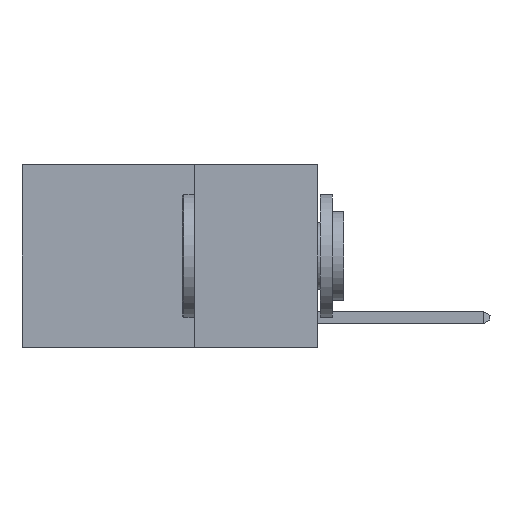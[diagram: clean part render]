
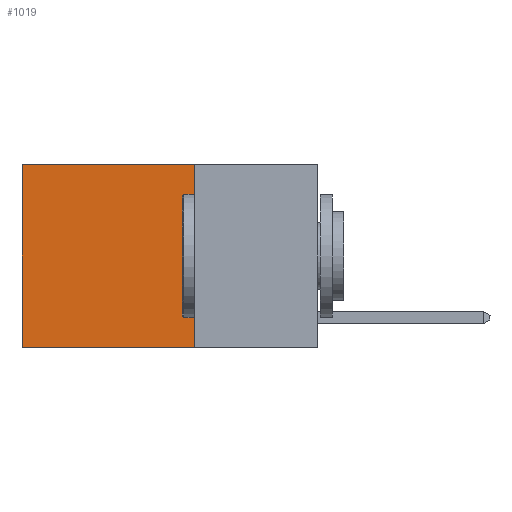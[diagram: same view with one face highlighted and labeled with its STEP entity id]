
A CAD part, left-side view. The second image highlights one B-rep face of the part: STEP entity #1019.
In plain terms, the highlighted planar face has unit normal (-1, 0, 0).
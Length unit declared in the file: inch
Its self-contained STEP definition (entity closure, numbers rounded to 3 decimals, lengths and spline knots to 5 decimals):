
#1019 = ADVANCED_FACE ( 'NONE', ( #9608 ), #25458, .F. ) ;
#2523 = VERTEX_POINT ( 'NONE', #10517 ) ;
#2994 = VECTOR ( 'NONE', #6338, 39.37008 ) ;
#3358 = AXIS2_PLACEMENT_3D ( 'NONE', #23123, #21051, #21425 ) ;
#3400 = LINE ( 'NONE', #19152, #12625 ) ;
#4655 = CARTESIAN_POINT ( 'NONE',  ( 0.2625, 0.25, 0. ) ) ;
#4751 = CARTESIAN_POINT ( 'NONE',  ( 0.2625, 0.6, 0. ) ) ;
#6338 = DIRECTION ( 'NONE',  ( 0., 1., 0. ) ) ;
#6712 = LINE ( 'NONE', #24162, #2994 ) ;
#6825 = DIRECTION ( 'NONE',  ( 0., 0., -1. ) ) ;
#8921 = VERTEX_POINT ( 'NONE', #10152 ) ;
#9272 = DIRECTION ( 'NONE',  ( 0., 0., -1. ) ) ;
#9608 = FACE_OUTER_BOUND ( 'NONE', #25697, .T. ) ;
#10152 = CARTESIAN_POINT ( 'NONE',  ( 0.2625, 0.6, -0.37 ) ) ;
#10384 = ORIENTED_EDGE ( 'NONE', *, *, #19988, .F. ) ;
#10517 = CARTESIAN_POINT ( 'NONE',  ( 0.2625, 0.6, 0. ) ) ;
#11798 = VECTOR ( 'NONE', #22477, 39.37008 ) ;
#12625 = VECTOR ( 'NONE', #9272, 39.37008 ) ;
#12741 = LINE ( 'NONE', #4655, #11798 ) ;
#12974 = EDGE_CURVE ( 'NONE', #18707, #8921, #6712, .T. ) ;
#14227 = ORIENTED_EDGE ( 'NONE', *, *, #12974, .F. ) ;
#14726 = CARTESIAN_POINT ( 'NONE',  ( 0.2625, 0.25, 0. ) ) ;
#17532 = EDGE_CURVE ( 'NONE', #22972, #2523, #12741, .T. ) ;
#18707 = VERTEX_POINT ( 'NONE', #22540 ) ;
#19152 = CARTESIAN_POINT ( 'NONE',  ( 0.2625, 0.25, 0. ) ) ;
#19363 = EDGE_CURVE ( 'NONE', #2523, #8921, #24150, .T. ) ;
#19988 = EDGE_CURVE ( 'NONE', #22972, #18707, #3400, .T. ) ;
#20817 = ORIENTED_EDGE ( 'NONE', *, *, #17532, .T. ) ;
#21051 = DIRECTION ( 'NONE',  ( 1., 0., 0. ) ) ;
#21425 = DIRECTION ( 'NONE',  ( 0., 0., -1. ) ) ;
#22477 = DIRECTION ( 'NONE',  ( 0., 1., 0. ) ) ;
#22540 = CARTESIAN_POINT ( 'NONE',  ( 0.2625, 0.25, -0.37 ) ) ;
#22957 = VECTOR ( 'NONE', #6825, 39.37008 ) ;
#22972 = VERTEX_POINT ( 'NONE', #14726 ) ;
#23123 = CARTESIAN_POINT ( 'NONE',  ( 0.2625, 0.25, 0. ) ) ;
#24150 = LINE ( 'NONE', #4751, #22957 ) ;
#24162 = CARTESIAN_POINT ( 'NONE',  ( 0.2625, 0.25, -0.37 ) ) ;
#24280 = ORIENTED_EDGE ( 'NONE', *, *, #19363, .T. ) ;
#25458 = PLANE ( 'NONE',  #3358 ) ;
#25697 = EDGE_LOOP ( 'NONE', ( #24280, #14227, #10384, #20817 ) ) ;
